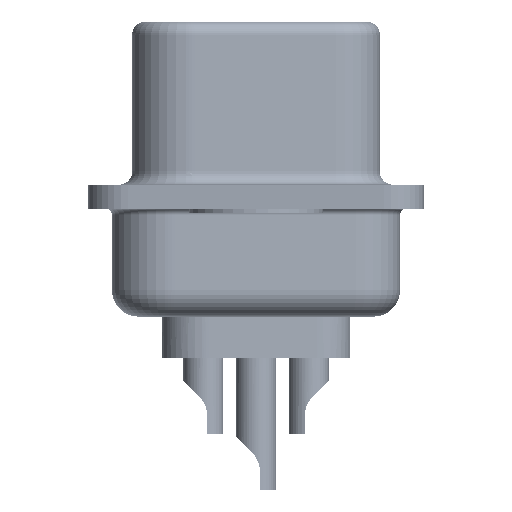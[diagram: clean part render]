
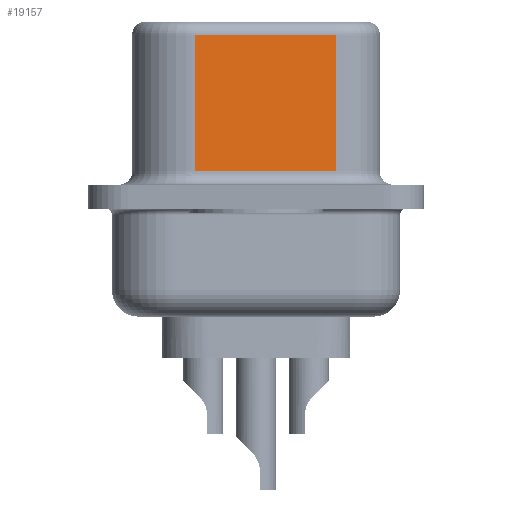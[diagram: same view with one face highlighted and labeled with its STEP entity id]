
A CAD part, left-side view. The second image highlights one B-rep face of the part: STEP entity #19157.
In plain terms, the highlighted planar face has unit normal (-0.985, -0.174, 0).
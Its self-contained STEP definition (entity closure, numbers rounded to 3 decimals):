
#3093 = CARTESIAN_POINT ( 'NONE',  ( 3.62, 2.293, 6.07 ) ) ;
#3366 = AXIS2_PLACEMENT_3D ( 'NONE', #18595, #12271, #26862 ) ;
#3636 = CARTESIAN_POINT ( 'NONE',  ( 3.62, 2.293, 6.57 ) ) ;
#4051 = DIRECTION ( 'NONE',  ( 0., 0., -1. ) ) ;
#5209 = DIRECTION ( 'NONE',  ( 0.174, -0.985, 0. ) ) ;
#5213 = LINE ( 'NONE', #21659, #19974 ) ;
#5975 = ORIENTED_EDGE ( 'NONE', *, *, #9090, .F. ) ;
#7283 = VECTOR ( 'NONE', #4051, 1000. ) ;
#8215 = VERTEX_POINT ( 'NONE', #3093 ) ;
#9090 = EDGE_CURVE ( 'NONE', #25329, #16169, #19281, .T. ) ;
#9417 = CARTESIAN_POINT ( 'NONE',  ( 4.551, -2.987, 0.95 ) ) ;
#9442 = LINE ( 'NONE', #18004, #22141 ) ;
#10343 = VECTOR ( 'NONE', #15073, 1000. ) ;
#11002 = DIRECTION ( 'NONE',  ( -0.174, 0.985, 0. ) ) ;
#12271 = DIRECTION ( 'NONE',  ( 0.985, 0.174, 0. ) ) ;
#12584 = EDGE_CURVE ( 'NONE', #8215, #22848, #12632, .T. ) ;
#12632 = LINE ( 'NONE', #3636, #7283 ) ;
#12824 = CARTESIAN_POINT ( 'NONE',  ( 4.551, -2.987, 6.57 ) ) ;
#13960 = ORIENTED_EDGE ( 'NONE', *, *, #12584, .T. ) ;
#13978 = FACE_OUTER_BOUND ( 'NONE', #19998, .T. ) ;
#15073 = DIRECTION ( 'NONE',  ( 0., 0., -1. ) ) ;
#16169 = VERTEX_POINT ( 'NONE', #9417 ) ;
#18004 = CARTESIAN_POINT ( 'NONE',  ( 4.551, -2.987, 0.95 ) ) ;
#18008 = CARTESIAN_POINT ( 'NONE',  ( 4.551, -2.987, 6.07 ) ) ;
#18595 = CARTESIAN_POINT ( 'NONE',  ( 4.551, -2.987, 6.57 ) ) ;
#18947 = CARTESIAN_POINT ( 'NONE',  ( 3.62, 2.293, 0.95 ) ) ;
#19157 = ADVANCED_FACE ( 'NONE', ( #13978 ), #24887, .F. ) ;
#19281 = LINE ( 'NONE', #12824, #10343 ) ;
#19711 = EDGE_CURVE ( 'NONE', #22848, #16169, #9442, .T. ) ;
#19974 = VECTOR ( 'NONE', #11002, 1000. ) ;
#19998 = EDGE_LOOP ( 'NONE', ( #5975, #22788, #13960, #26933 ) ) ;
#20933 = EDGE_CURVE ( 'NONE', #25329, #8215, #5213, .T. ) ;
#21659 = CARTESIAN_POINT ( 'NONE',  ( 4.551, -2.987, 6.07 ) ) ;
#22141 = VECTOR ( 'NONE', #5209, 1000. ) ;
#22788 = ORIENTED_EDGE ( 'NONE', *, *, #20933, .T. ) ;
#22848 = VERTEX_POINT ( 'NONE', #18947 ) ;
#24887 = PLANE ( 'NONE',  #3366 ) ;
#25329 = VERTEX_POINT ( 'NONE', #18008 ) ;
#26862 = DIRECTION ( 'NONE',  ( -0.174, 0.985, 0. ) ) ;
#26933 = ORIENTED_EDGE ( 'NONE', *, *, #19711, .T. ) ;
